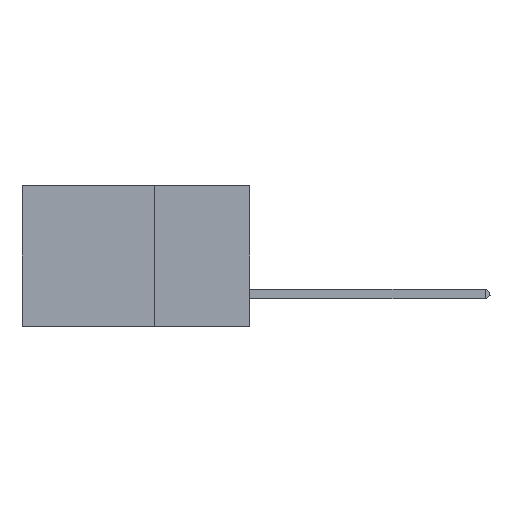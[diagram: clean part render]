
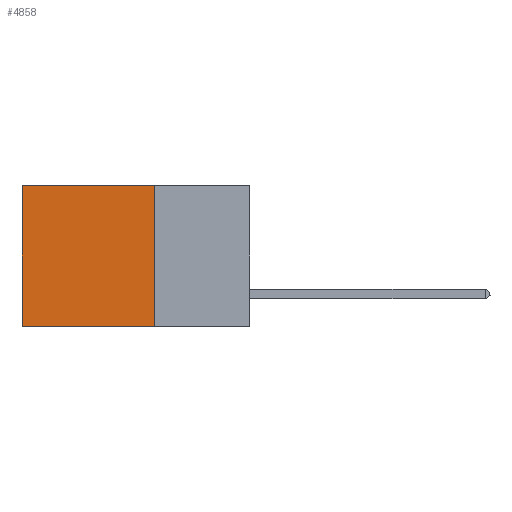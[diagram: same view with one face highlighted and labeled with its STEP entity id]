
A CAD part, left-side view. The second image highlights one B-rep face of the part: STEP entity #4858.
In plain terms, the highlighted planar face has unit normal (-1, 0, 0).
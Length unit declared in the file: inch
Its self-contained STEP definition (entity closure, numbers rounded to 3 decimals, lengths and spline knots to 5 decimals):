
#36 = EDGE_CURVE ( 'NONE', #10633, #16801, #10236, .T. ) ;
#382 = LINE ( 'NONE', #4241, #2240 ) ;
#1472 = VERTEX_POINT ( 'NONE', #10228 ) ;
#1603 = DIRECTION ( 'NONE',  ( 0., 0., -1. ) ) ;
#2240 = VECTOR ( 'NONE', #4309, 39.37008 ) ;
#2411 = CARTESIAN_POINT ( 'NONE',  ( 0.2875, 0.25, 0. ) ) ;
#3524 = EDGE_CURVE ( 'NONE', #16801, #1472, #382, .T. ) ;
#3753 = AXIS2_PLACEMENT_3D ( 'NONE', #9248, #6258, #7745 ) ;
#3799 = LINE ( 'NONE', #5041, #10076 ) ;
#4241 = CARTESIAN_POINT ( 'NONE',  ( 0.2875, 0.25, -0.37 ) ) ;
#4309 = DIRECTION ( 'NONE',  ( 0., 1., 0. ) ) ;
#4858 = ADVANCED_FACE ( 'NONE', ( #16109 ), #14867, .F. ) ;
#5041 = CARTESIAN_POINT ( 'NONE',  ( 0.2875, 0.25, 0. ) ) ;
#5047 = VECTOR ( 'NONE', #1603, 39.37008 ) ;
#5918 = ORIENTED_EDGE ( 'NONE', *, *, #8059, .T. ) ;
#5937 = ORIENTED_EDGE ( 'NONE', *, *, #36, .F. ) ;
#6258 = DIRECTION ( 'NONE',  ( 1., 0., 0. ) ) ;
#6886 = EDGE_LOOP ( 'NONE', ( #8126, #17245, #5937, #5918 ) ) ;
#7472 = VECTOR ( 'NONE', #17640, 39.37008 ) ;
#7745 = DIRECTION ( 'NONE',  ( 0., 0., -1. ) ) ;
#7922 = VERTEX_POINT ( 'NONE', #8680 ) ;
#8059 = EDGE_CURVE ( 'NONE', #10633, #7922, #3799, .T. ) ;
#8126 = ORIENTED_EDGE ( 'NONE', *, *, #11590, .T. ) ;
#8680 = CARTESIAN_POINT ( 'NONE',  ( 0.2875, 0.6, 0. ) ) ;
#9248 = CARTESIAN_POINT ( 'NONE',  ( 0.2875, 0.25, 0. ) ) ;
#10076 = VECTOR ( 'NONE', #15084, 39.37008 ) ;
#10228 = CARTESIAN_POINT ( 'NONE',  ( 0.2875, 0.6, -0.37 ) ) ;
#10236 = LINE ( 'NONE', #10909, #5047 ) ;
#10633 = VERTEX_POINT ( 'NONE', #2411 ) ;
#10637 = LINE ( 'NONE', #16188, #7472 ) ;
#10909 = CARTESIAN_POINT ( 'NONE',  ( 0.2875, 0.25, 0. ) ) ;
#11590 = EDGE_CURVE ( 'NONE', #7922, #1472, #10637, .T. ) ;
#14867 = PLANE ( 'NONE',  #3753 ) ;
#15084 = DIRECTION ( 'NONE',  ( 0., 1., 0. ) ) ;
#16109 = FACE_OUTER_BOUND ( 'NONE', #6886, .T. ) ;
#16188 = CARTESIAN_POINT ( 'NONE',  ( 0.2875, 0.6, 0. ) ) ;
#16210 = CARTESIAN_POINT ( 'NONE',  ( 0.2875, 0.25, -0.37 ) ) ;
#16801 = VERTEX_POINT ( 'NONE', #16210 ) ;
#17245 = ORIENTED_EDGE ( 'NONE', *, *, #3524, .F. ) ;
#17640 = DIRECTION ( 'NONE',  ( 0., 0., -1. ) ) ;
